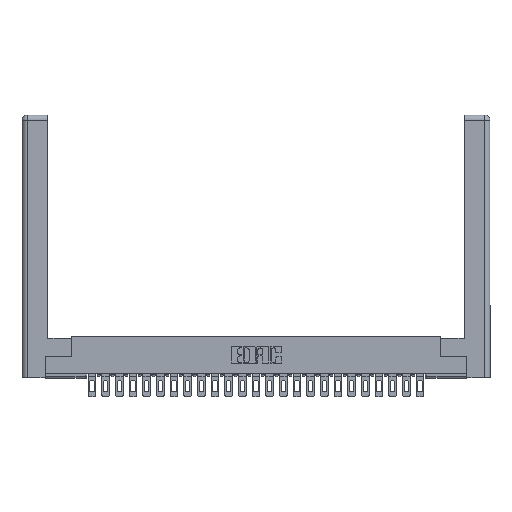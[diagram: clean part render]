
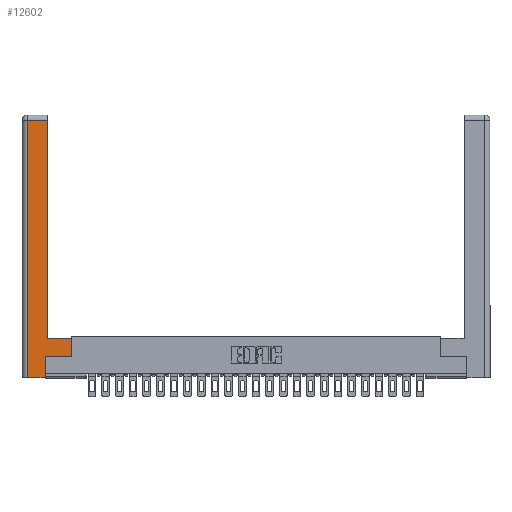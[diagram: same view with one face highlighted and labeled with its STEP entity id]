
A CAD part, top view. The second image highlights one B-rep face of the part: STEP entity #12602.
In plain terms, the highlighted planar face has unit normal (0, 0, 1).
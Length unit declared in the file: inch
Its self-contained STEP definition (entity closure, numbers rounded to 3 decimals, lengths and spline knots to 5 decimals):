
#49 = LINE ( 'NONE', #16648, #14007 ) ;
#87 = VECTOR ( 'NONE', #11655, 39.37008 ) ;
#603 = ORIENTED_EDGE ( 'NONE', *, *, #787, .T. ) ;
#787 = EDGE_CURVE ( 'NONE', #21648, #21830, #23183, .T. ) ;
#1272 = EDGE_CURVE ( 'NONE', #21698, #1626, #11788, .T. ) ;
#1322 = CARTESIAN_POINT ( 'NONE',  ( 0.565, 0.245, 0. ) ) ;
#1498 = EDGE_CURVE ( 'NONE', #25579, #16860, #49, .T. ) ;
#1626 = VERTEX_POINT ( 'NONE', #19129 ) ;
#2334 = CARTESIAN_POINT ( 'NONE',  ( 0.0615, 2.94, 0. ) ) ;
#3170 = EDGE_CURVE ( 'NONE', #1626, #17154, #10694, .T. ) ;
#3976 = LINE ( 'NONE', #24283, #87 ) ;
#3978 = DIRECTION ( 'NONE',  ( 0., 1., 0. ) ) ;
#4177 = VERTEX_POINT ( 'NONE', #2334 ) ;
#4184 = PLANE ( 'NONE',  #22572 ) ;
#4628 = VECTOR ( 'NONE', #10033, 39.37008 ) ;
#7119 = ORIENTED_EDGE ( 'NONE', *, *, #25709, .T. ) ;
#7228 = ORIENTED_EDGE ( 'NONE', *, *, #25672, .T. ) ;
#8325 = DIRECTION ( 'NONE',  ( 1., 0., 0. ) ) ;
#8514 = ORIENTED_EDGE ( 'NONE', *, *, #1498, .T. ) ;
#8546 = VECTOR ( 'NONE', #22230, 39.37008 ) ;
#8861 = LINE ( 'NONE', #18952, #26085 ) ;
#9224 = VECTOR ( 'NONE', #3978, 39.37008 ) ;
#10033 = DIRECTION ( 'NONE',  ( 0., 1., 0. ) ) ;
#10694 = LINE ( 'NONE', #22837, #14244 ) ;
#11655 = DIRECTION ( 'NONE',  ( -1., 0., 0. ) ) ;
#11788 = LINE ( 'NONE', #1322, #8546 ) ;
#12602 = ADVANCED_FACE ( 'NONE', ( #13647 ), #4184, .F. ) ;
#13647 = FACE_OUTER_BOUND ( 'NONE', #21387, .T. ) ;
#13765 = ORIENTED_EDGE ( 'NONE', *, *, #1272, .T. ) ;
#14007 = VECTOR ( 'NONE', #8325, 39.37008 ) ;
#14152 = LINE ( 'NONE', #21309, #26859 ) ;
#14244 = VECTOR ( 'NONE', #20483, 39.37008 ) ;
#14469 = CARTESIAN_POINT ( 'NONE',  ( 0.265, 0., 0. ) ) ;
#14611 = DIRECTION ( 'NONE',  ( -1., 0., 0. ) ) ;
#15103 = DIRECTION ( 'NONE',  ( -1., 0., 0. ) ) ;
#16648 = CARTESIAN_POINT ( 'NONE',  ( 0.265, 0., 0. ) ) ;
#16650 = DIRECTION ( 'NONE',  ( 0., -1., 0. ) ) ;
#16860 = VERTEX_POINT ( 'NONE', #14469 ) ;
#17154 = VERTEX_POINT ( 'NONE', #17667 ) ;
#17179 = EDGE_CURVE ( 'NONE', #17154, #21648, #3976, .T. ) ;
#17667 = CARTESIAN_POINT ( 'NONE',  ( 0.565, 0.45, 0. ) ) ;
#17850 = ORIENTED_EDGE ( 'NONE', *, *, #17179, .T. ) ;
#18138 = CARTESIAN_POINT ( 'NONE',  ( 0.0615, 0., 0. ) ) ;
#18319 = CARTESIAN_POINT ( 'NONE',  ( 0.265, 0.245, 0. ) ) ;
#18465 = CARTESIAN_POINT ( 'NONE',  ( 0., 0., 0. ) ) ;
#18952 = CARTESIAN_POINT ( 'NONE',  ( 0.0615, 0., 0. ) ) ;
#19129 = CARTESIAN_POINT ( 'NONE',  ( 0.565, 0.245, 0. ) ) ;
#19448 = CARTESIAN_POINT ( 'NONE',  ( 0.265, 0.245, 0. ) ) ;
#19884 = CARTESIAN_POINT ( 'NONE',  ( 0.295, 2.94, 0. ) ) ;
#20483 = DIRECTION ( 'NONE',  ( 0., 1., 0. ) ) ;
#20722 = ORIENTED_EDGE ( 'NONE', *, *, #3170, .T. ) ;
#20884 = CARTESIAN_POINT ( 'NONE',  ( 0.295, 3., 0. ) ) ;
#20917 = DIRECTION ( 'NONE',  ( 0., 0., -1. ) ) ;
#20969 = EDGE_CURVE ( 'NONE', #21830, #4177, #14152, .T. ) ;
#21309 = CARTESIAN_POINT ( 'NONE',  ( 0.0615, 2.94, 0. ) ) ;
#21387 = EDGE_LOOP ( 'NONE', ( #603, #23769, #7119, #8514, #7228, #13765, #20722, #17850 ) ) ;
#21648 = VERTEX_POINT ( 'NONE', #23338 ) ;
#21698 = VERTEX_POINT ( 'NONE', #19448 ) ;
#21830 = VERTEX_POINT ( 'NONE', #19884 ) ;
#22230 = DIRECTION ( 'NONE',  ( 1., 0., 0. ) ) ;
#22526 = LINE ( 'NONE', #18319, #4628 ) ;
#22572 = AXIS2_PLACEMENT_3D ( 'NONE', #18465, #20917, #14611 ) ;
#22837 = CARTESIAN_POINT ( 'NONE',  ( 0.565, 0.45, 0. ) ) ;
#23183 = LINE ( 'NONE', #20884, #9224 ) ;
#23338 = CARTESIAN_POINT ( 'NONE',  ( 0.295, 0.45, 0. ) ) ;
#23769 = ORIENTED_EDGE ( 'NONE', *, *, #20969, .T. ) ;
#24283 = CARTESIAN_POINT ( 'NONE',  ( 0.295, 0.45, 0. ) ) ;
#25579 = VERTEX_POINT ( 'NONE', #18138 ) ;
#25672 = EDGE_CURVE ( 'NONE', #16860, #21698, #22526, .T. ) ;
#25709 = EDGE_CURVE ( 'NONE', #4177, #25579, #8861, .T. ) ;
#26085 = VECTOR ( 'NONE', #16650, 39.37008 ) ;
#26859 = VECTOR ( 'NONE', #15103, 39.37008 ) ;
